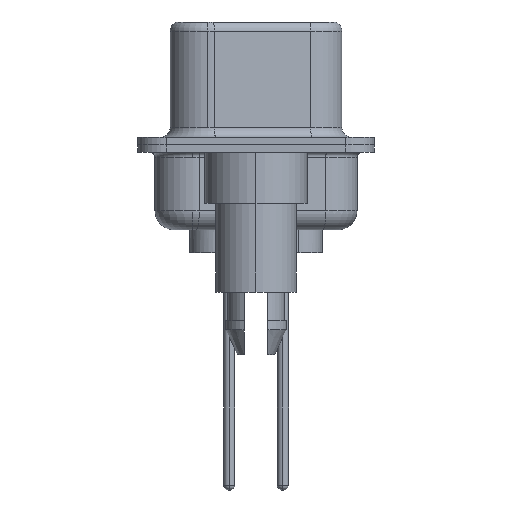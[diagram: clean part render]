
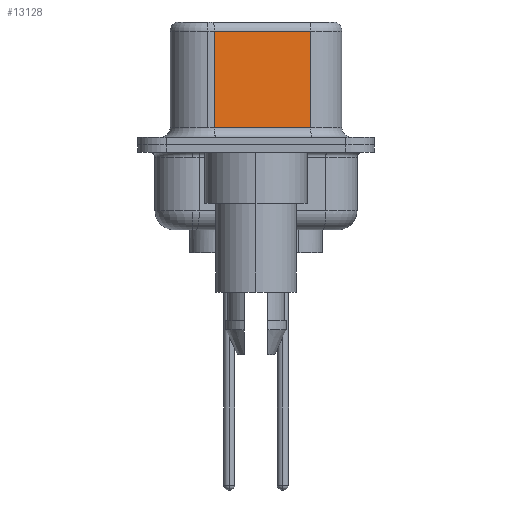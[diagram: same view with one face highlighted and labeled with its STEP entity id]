
A CAD part, left-side view. The second image highlights one B-rep face of the part: STEP entity #13128.
In plain terms, the highlighted planar face has unit normal (-0.985, -0.174, 0).
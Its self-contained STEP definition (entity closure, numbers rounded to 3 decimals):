
#741 = DIRECTION ( 'NONE',  ( 0.985, 0.174, 0. ) ) ;
#808 = CARTESIAN_POINT ( 'NONE',  ( 3.655, 2.203, 6.52 ) ) ;
#916 = CARTESIAN_POINT ( 'NONE',  ( 4.555, -2.897, 6.52 ) ) ;
#1926 = VECTOR ( 'NONE', #14504, 1000. ) ;
#2391 = CARTESIAN_POINT ( 'NONE',  ( 4.555, -2.897, 6.02 ) ) ;
#2864 = VERTEX_POINT ( 'NONE', #11202 ) ;
#3359 = PLANE ( 'NONE',  #5671 ) ;
#3932 = VERTEX_POINT ( 'NONE', #8453 ) ;
#4163 = VERTEX_POINT ( 'NONE', #11402 ) ;
#5212 = DIRECTION ( 'NONE',  ( -0.174, 0.985, 0. ) ) ;
#5671 = AXIS2_PLACEMENT_3D ( 'NONE', #9100, #741, #6161 ) ;
#6161 = DIRECTION ( 'NONE',  ( -0.174, 0.985, 0. ) ) ;
#6347 = LINE ( 'NONE', #916, #13212 ) ;
#6350 = ORIENTED_EDGE ( 'NONE', *, *, #10707, .T. ) ;
#7186 = ORIENTED_EDGE ( 'NONE', *, *, #17767, .F. ) ;
#8028 = ORIENTED_EDGE ( 'NONE', *, *, #11155, .T. ) ;
#8453 = CARTESIAN_POINT ( 'NONE',  ( 4.555, -2.897, 6.02 ) ) ;
#8726 = ORIENTED_EDGE ( 'NONE', *, *, #14532, .T. ) ;
#9100 = CARTESIAN_POINT ( 'NONE',  ( 4.555, -2.897, 6.52 ) ) ;
#10707 = EDGE_CURVE ( 'NONE', #2864, #11304, #15867, .T. ) ;
#11060 = CARTESIAN_POINT ( 'NONE',  ( 4.555, -2.897, 0.9 ) ) ;
#11155 = EDGE_CURVE ( 'NONE', #3932, #2864, #14736, .T. ) ;
#11202 = CARTESIAN_POINT ( 'NONE',  ( 3.655, 2.203, 6.02 ) ) ;
#11304 = VERTEX_POINT ( 'NONE', #12379 ) ;
#11402 = CARTESIAN_POINT ( 'NONE',  ( 4.555, -2.897, 0.9 ) ) ;
#11454 = FACE_OUTER_BOUND ( 'NONE', #12602, .T. ) ;
#11991 = VECTOR ( 'NONE', #5212, 1000. ) ;
#12320 = LINE ( 'NONE', #11060, #15163 ) ;
#12379 = CARTESIAN_POINT ( 'NONE',  ( 3.655, 2.203, 0.9 ) ) ;
#12602 = EDGE_LOOP ( 'NONE', ( #7186, #8028, #6350, #8726 ) ) ;
#13128 = ADVANCED_FACE ( 'NONE', ( #11454 ), #3359, .F. ) ;
#13212 = VECTOR ( 'NONE', #14712, 1000. ) ;
#14504 = DIRECTION ( 'NONE',  ( 0., 0., -1. ) ) ;
#14532 = EDGE_CURVE ( 'NONE', #11304, #4163, #12320, .T. ) ;
#14712 = DIRECTION ( 'NONE',  ( 0., 0., -1. ) ) ;
#14736 = LINE ( 'NONE', #2391, #11991 ) ;
#15163 = VECTOR ( 'NONE', #16585, 1000. ) ;
#15867 = LINE ( 'NONE', #808, #1926 ) ;
#16585 = DIRECTION ( 'NONE',  ( 0.174, -0.985, 0. ) ) ;
#17767 = EDGE_CURVE ( 'NONE', #3932, #4163, #6347, .T. ) ;
